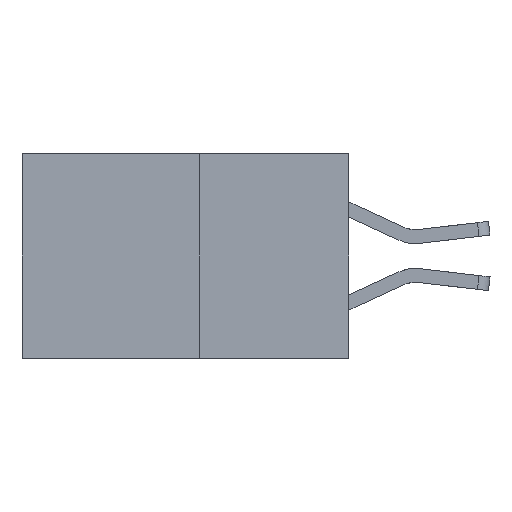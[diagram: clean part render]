
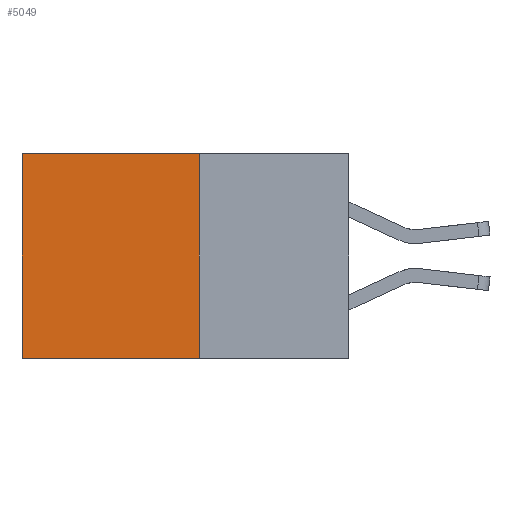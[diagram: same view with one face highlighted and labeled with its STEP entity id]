
A CAD part, left-side view. The second image highlights one B-rep face of the part: STEP entity #5049.
In plain terms, the highlighted planar face has unit normal (-1, 0, 0).
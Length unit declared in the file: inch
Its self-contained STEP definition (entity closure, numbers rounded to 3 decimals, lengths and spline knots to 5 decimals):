
#328 = DIRECTION ( 'NONE',  ( 0., 0., -1. ) ) ;
#956 = VECTOR ( 'NONE', #2097, 39.37008 ) ;
#1166 = ORIENTED_EDGE ( 'NONE', *, *, #11587, .F. ) ;
#1323 = CARTESIAN_POINT ( 'NONE',  ( 0.277, 0.27, 0. ) ) ;
#1365 = AXIS2_PLACEMENT_3D ( 'NONE', #9905, #9571, #9247 ) ;
#1456 = CARTESIAN_POINT ( 'NONE',  ( 0.277, 0.59, 0. ) ) ;
#2097 = DIRECTION ( 'NONE',  ( 0., 0., -1. ) ) ;
#2270 = EDGE_CURVE ( 'NONE', #11681, #11932, #10480, .T. ) ;
#2303 = VECTOR ( 'NONE', #3211, 39.37008 ) ;
#2533 = VERTEX_POINT ( 'NONE', #5425 ) ;
#2948 = ORIENTED_EDGE ( 'NONE', *, *, #2270, .T. ) ;
#3211 = DIRECTION ( 'NONE',  ( 0., 1., 0. ) ) ;
#3219 = CARTESIAN_POINT ( 'NONE',  ( 0.277, 0.27, -0.37 ) ) ;
#3298 = CARTESIAN_POINT ( 'NONE',  ( 0.277, 0.27, -0.37 ) ) ;
#3785 = CARTESIAN_POINT ( 'NONE',  ( 0.277, 0.59, -0.37 ) ) ;
#4294 = VECTOR ( 'NONE', #328, 39.37008 ) ;
#4666 = VECTOR ( 'NONE', #6205, 39.37008 ) ;
#5049 = ADVANCED_FACE ( 'NONE', ( #5567 ), #9937, .F. ) ;
#5425 = CARTESIAN_POINT ( 'NONE',  ( 0.277, 0.27, 0. ) ) ;
#5567 = FACE_OUTER_BOUND ( 'NONE', #8247, .T. ) ;
#6205 = DIRECTION ( 'NONE',  ( 0., 1., 0. ) ) ;
#6342 = CARTESIAN_POINT ( 'NONE',  ( 0.277, 0.27, -0.37 ) ) ;
#6573 = EDGE_CURVE ( 'NONE', #2533, #11681, #9858, .T. ) ;
#6612 = ORIENTED_EDGE ( 'NONE', *, *, #8627, .F. ) ;
#7197 = LINE ( 'NONE', #3298, #4666 ) ;
#7871 = ORIENTED_EDGE ( 'NONE', *, *, #6573, .T. ) ;
#8247 = EDGE_LOOP ( 'NONE', ( #2948, #6612, #1166, #7871 ) ) ;
#8627 = EDGE_CURVE ( 'NONE', #11731, #11932, #7197, .T. ) ;
#9247 = DIRECTION ( 'NONE',  ( 0., 0., -1. ) ) ;
#9571 = DIRECTION ( 'NONE',  ( 1., 0., 0. ) ) ;
#9858 = LINE ( 'NONE', #1323, #2303 ) ;
#9905 = CARTESIAN_POINT ( 'NONE',  ( 0.277, 0.27, -0.37 ) ) ;
#9937 = PLANE ( 'NONE',  #1365 ) ;
#10480 = LINE ( 'NONE', #3785, #956 ) ;
#11587 = EDGE_CURVE ( 'NONE', #2533, #11731, #11824, .T. ) ;
#11681 = VERTEX_POINT ( 'NONE', #1456 ) ;
#11731 = VERTEX_POINT ( 'NONE', #6342 ) ;
#11824 = LINE ( 'NONE', #3219, #4294 ) ;
#11932 = VERTEX_POINT ( 'NONE', #12255 ) ;
#12255 = CARTESIAN_POINT ( 'NONE',  ( 0.277, 0.59, -0.37 ) ) ;
